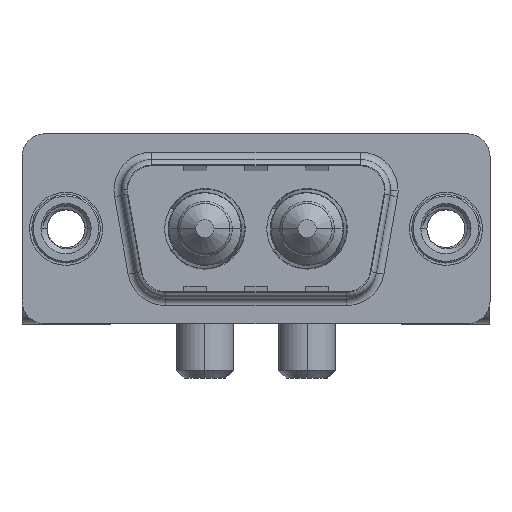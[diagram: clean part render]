
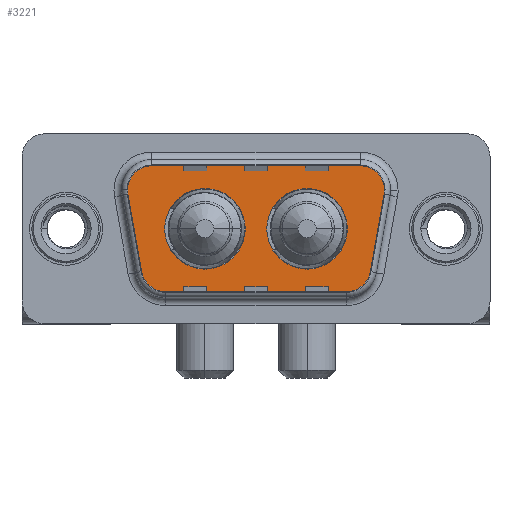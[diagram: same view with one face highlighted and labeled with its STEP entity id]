
A CAD part, top view. The second image highlights one B-rep face of the part: STEP entity #3221.
In plain terms, the highlighted planar face has unit normal (0, 0, 1).
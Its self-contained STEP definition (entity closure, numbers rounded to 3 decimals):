
#187 = DIRECTION ( 'NONE',  ( 1., 0., 0. ) ) ;
#350 = CIRCLE ( 'NONE', #2178, 2.65 ) ;
#510 = ORIENTED_EDGE ( 'NONE', *, *, #7918, .T. ) ;
#668 = VERTEX_POINT ( 'NONE', #9702 ) ;
#802 = CARTESIAN_POINT ( 'NONE',  ( 13.21, 0., 0. ) ) ;
#815 = AXIS2_PLACEMENT_3D ( 'NONE', #6807, #5510, #8863 ) ;
#968 = VERTEX_POINT ( 'NONE', #3896 ) ;
#1190 = FACE_BOUND ( 'NONE', #9778, .T. ) ;
#1274 = VERTEX_POINT ( 'NONE', #4684 ) ;
#1280 = ORIENTED_EDGE ( 'NONE', *, *, #4547, .F. ) ;
#1512 = CARTESIAN_POINT ( 'NONE',  ( 20.511, -3.247, 0. ) ) ;
#1530 = LINE ( 'NONE', #4518, #11005 ) ;
#1632 = ORIENTED_EDGE ( 'NONE', *, *, #5015, .T. ) ;
#1717 = EDGE_LOOP ( 'NONE', ( #4952, #3962 ) ) ;
#1904 = DIRECTION ( 'NONE',  ( 0., 0., 1. ) ) ;
#1938 = CARTESIAN_POINT ( 'NONE',  ( 3.466, 2.553, 0. ) ) ;
#1983 = CARTESIAN_POINT ( 'NONE',  ( 9.14, 0., 0. ) ) ;
#2006 = VECTOR ( 'NONE', #7279, 1000. ) ;
#2105 = CARTESIAN_POINT ( 'NONE',  ( 6.49, 0., 0. ) ) ;
#2178 = AXIS2_PLACEMENT_3D ( 'NONE', #4110, #7251, #9371 ) ;
#2471 = VERTEX_POINT ( 'NONE', #9117 ) ;
#2723 = CARTESIAN_POINT ( 'NONE',  ( 19.564, 4.9, 0. ) ) ;
#2859 = EDGE_CURVE ( 'NONE', #3898, #968, #11094, .T. ) ;
#2924 = LINE ( 'NONE', #1938, #2006 ) ;
#2959 = ORIENTED_EDGE ( 'NONE', *, *, #12360, .F. ) ;
#3020 = CARTESIAN_POINT ( 'NONE',  ( 19.564, 2.9, 0. ) ) ;
#3098 = DIRECTION ( 'NONE',  ( 0., 0., 1. ) ) ;
#3185 = PLANE ( 'NONE',  #10825 ) ;
#3221 = ADVANCED_FACE ( 'NONE', ( #5598, #1190, #7676 ), #3185, .T. ) ;
#3478 = DIRECTION ( 'NONE',  ( -1., 0., 0. ) ) ;
#3725 = CIRCLE ( 'NONE', #5078, 2.65 ) ;
#3896 = CARTESIAN_POINT ( 'NONE',  ( 21.534, 2.553, 0. ) ) ;
#3898 = VERTEX_POINT ( 'NONE', #1512 ) ;
#3962 = ORIENTED_EDGE ( 'NONE', *, *, #5871, .F. ) ;
#4110 = CARTESIAN_POINT ( 'NONE',  ( 9.14, 0., 0. ) ) ;
#4177 = CIRCLE ( 'NONE', #12139, 2.65 ) ;
#4190 = CARTESIAN_POINT ( 'NONE',  ( 18.541, -2.9, 0. ) ) ;
#4235 = DIRECTION ( 'NONE',  ( -1., 0., 0. ) ) ;
#4236 = CARTESIAN_POINT ( 'NONE',  ( 11.79, 0., 0. ) ) ;
#4260 = ORIENTED_EDGE ( 'NONE', *, *, #10070, .T. ) ;
#4332 = EDGE_CURVE ( 'NONE', #9857, #13498, #8963, .T. ) ;
#4518 = CARTESIAN_POINT ( 'NONE',  ( 6.459, -4.9, 0. ) ) ;
#4547 = EDGE_CURVE ( 'NONE', #7756, #9328, #11451, .T. ) ;
#4684 = CARTESIAN_POINT ( 'NONE',  ( 3.466, 2.553, 0. ) ) ;
#4914 = VECTOR ( 'NONE', #9812, 1000. ) ;
#4952 = ORIENTED_EDGE ( 'NONE', *, *, #5518, .F. ) ;
#5015 = EDGE_CURVE ( 'NONE', #11689, #9857, #7166, .T. ) ;
#5078 = AXIS2_PLACEMENT_3D ( 'NONE', #11537, #7283, #12685 ) ;
#5082 = AXIS2_PLACEMENT_3D ( 'NONE', #4190, #8540, #12585 ) ;
#5172 = VECTOR ( 'NONE', #3478, 1000. ) ;
#5215 = DIRECTION ( 'NONE',  ( 1., 0., 0. ) ) ;
#5285 = VERTEX_POINT ( 'NONE', #7796 ) ;
#5335 = AXIS2_PLACEMENT_3D ( 'NONE', #3020, #3098, #4235 ) ;
#5404 = CARTESIAN_POINT ( 'NONE',  ( 21.534, 2.553, 0. ) ) ;
#5510 = DIRECTION ( 'NONE',  ( 0., 0., 1. ) ) ;
#5518 = EDGE_CURVE ( 'NONE', #12293, #6815, #3725, .T. ) ;
#5598 = FACE_BOUND ( 'NONE', #1717, .T. ) ;
#5695 = CARTESIAN_POINT ( 'NONE',  ( 5.436, 4.9, 0. ) ) ;
#5826 = CIRCLE ( 'NONE', #13096, 2. ) ;
#5871 = EDGE_CURVE ( 'NONE', #6815, #12293, #4177, .T. ) ;
#5915 = CARTESIAN_POINT ( 'NONE',  ( 21.564, 2.9, 0. ) ) ;
#6015 = ORIENTED_EDGE ( 'NONE', *, *, #11079, .T. ) ;
#6583 = ORIENTED_EDGE ( 'NONE', *, *, #8227, .T. ) ;
#6742 = AXIS2_PLACEMENT_3D ( 'NONE', #8549, #12884, #10600 ) ;
#6807 = CARTESIAN_POINT ( 'NONE',  ( 6.459, -2.9, 0. ) ) ;
#6815 = VERTEX_POINT ( 'NONE', #802 ) ;
#6961 = CIRCLE ( 'NONE', #815, 2. ) ;
#7166 = CIRCLE ( 'NONE', #5335, 2. ) ;
#7251 = DIRECTION ( 'NONE',  ( 0., 0., 1. ) ) ;
#7279 = DIRECTION ( 'NONE',  ( 0.174, -0.985, 0. ) ) ;
#7283 = DIRECTION ( 'NONE',  ( 0., 0., 1. ) ) ;
#7676 = FACE_OUTER_BOUND ( 'NONE', #9151, .T. ) ;
#7756 = VERTEX_POINT ( 'NONE', #4236 ) ;
#7784 = ORIENTED_EDGE ( 'NONE', *, *, #4332, .T. ) ;
#7796 = CARTESIAN_POINT ( 'NONE',  ( 6.459, -4.9, 0. ) ) ;
#7822 = CIRCLE ( 'NONE', #5082, 2. ) ;
#7855 = DIRECTION ( 'NONE',  ( 1., 0., 0. ) ) ;
#7918 = EDGE_CURVE ( 'NONE', #2471, #5285, #6961, .T. ) ;
#8227 = EDGE_CURVE ( 'NONE', #968, #11689, #13319, .T. ) ;
#8540 = DIRECTION ( 'NONE',  ( 0., 0., 1. ) ) ;
#8549 = CARTESIAN_POINT ( 'NONE',  ( 19.564, 2.9, 0. ) ) ;
#8707 = ORIENTED_EDGE ( 'NONE', *, *, #12915, .T. ) ;
#8863 = DIRECTION ( 'NONE',  ( -1., 0., 0. ) ) ;
#8911 = CARTESIAN_POINT ( 'NONE',  ( 15.86, 0., 0. ) ) ;
#8928 = DIRECTION ( 'NONE',  ( 1., 0., 0. ) ) ;
#8963 = LINE ( 'NONE', #12166, #5172 ) ;
#9117 = CARTESIAN_POINT ( 'NONE',  ( 4.489, -3.247, 0. ) ) ;
#9151 = EDGE_LOOP ( 'NONE', ( #10310, #12759, #6583, #1632, #7784, #8707, #4260, #510, #6015 ) ) ;
#9304 = CARTESIAN_POINT ( 'NONE',  ( 18.51, 0., 0. ) ) ;
#9328 = VERTEX_POINT ( 'NONE', #2105 ) ;
#9371 = DIRECTION ( 'NONE',  ( 1., 0., 0. ) ) ;
#9702 = CARTESIAN_POINT ( 'NONE',  ( 18.541, -4.9, 0. ) ) ;
#9778 = EDGE_LOOP ( 'NONE', ( #1280, #2959 ) ) ;
#9812 = DIRECTION ( 'NONE',  ( 0.174, 0.985, 0. ) ) ;
#9857 = VERTEX_POINT ( 'NONE', #2723 ) ;
#9869 = DIRECTION ( 'NONE',  ( 0., 0., 1. ) ) ;
#10070 = EDGE_CURVE ( 'NONE', #1274, #2471, #2924, .T. ) ;
#10310 = ORIENTED_EDGE ( 'NONE', *, *, #13764, .T. ) ;
#10600 = DIRECTION ( 'NONE',  ( -1., 0., 0. ) ) ;
#10774 = AXIS2_PLACEMENT_3D ( 'NONE', #1983, #1904, #11573 ) ;
#10825 = AXIS2_PLACEMENT_3D ( 'NONE', #12931, #9869, #187 ) ;
#11005 = VECTOR ( 'NONE', #8928, 1000. ) ;
#11079 = EDGE_CURVE ( 'NONE', #5285, #668, #1530, .T. ) ;
#11094 = LINE ( 'NONE', #5404, #4914 ) ;
#11451 = CIRCLE ( 'NONE', #10774, 2.65 ) ;
#11537 = CARTESIAN_POINT ( 'NONE',  ( 15.86, 0., 0. ) ) ;
#11573 = DIRECTION ( 'NONE',  ( 1., 0., 0. ) ) ;
#11689 = VERTEX_POINT ( 'NONE', #5915 ) ;
#12139 = AXIS2_PLACEMENT_3D ( 'NONE', #8911, #13526, #7855 ) ;
#12166 = CARTESIAN_POINT ( 'NONE',  ( 5.436, 4.9, 0. ) ) ;
#12293 = VERTEX_POINT ( 'NONE', #9304 ) ;
#12360 = EDGE_CURVE ( 'NONE', #9328, #7756, #350, .T. ) ;
#12585 = DIRECTION ( 'NONE',  ( 1., 0., 0. ) ) ;
#12685 = DIRECTION ( 'NONE',  ( 1., 0., 0. ) ) ;
#12695 = DIRECTION ( 'NONE',  ( 0., 0., 1. ) ) ;
#12759 = ORIENTED_EDGE ( 'NONE', *, *, #2859, .T. ) ;
#12884 = DIRECTION ( 'NONE',  ( 0., 0., 1. ) ) ;
#12915 = EDGE_CURVE ( 'NONE', #13498, #1274, #5826, .T. ) ;
#12931 = CARTESIAN_POINT ( 'NONE',  ( 18.541, -2.9, 0. ) ) ;
#13096 = AXIS2_PLACEMENT_3D ( 'NONE', #13833, #12695, #5215 ) ;
#13319 = CIRCLE ( 'NONE', #6742, 2. ) ;
#13498 = VERTEX_POINT ( 'NONE', #5695 ) ;
#13526 = DIRECTION ( 'NONE',  ( 0., 0., 1. ) ) ;
#13764 = EDGE_CURVE ( 'NONE', #668, #3898, #7822, .T. ) ;
#13833 = CARTESIAN_POINT ( 'NONE',  ( 5.436, 2.9, 0. ) ) ;
